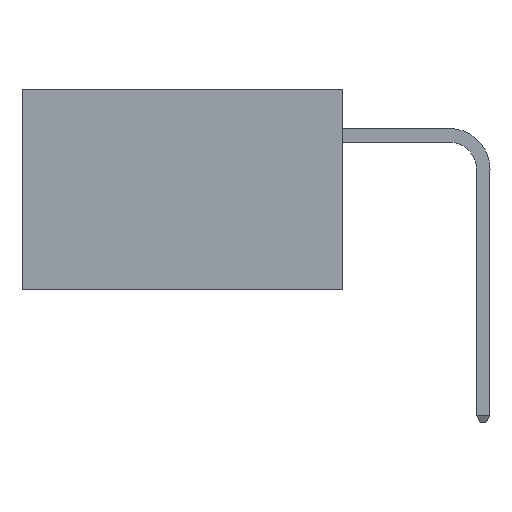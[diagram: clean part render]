
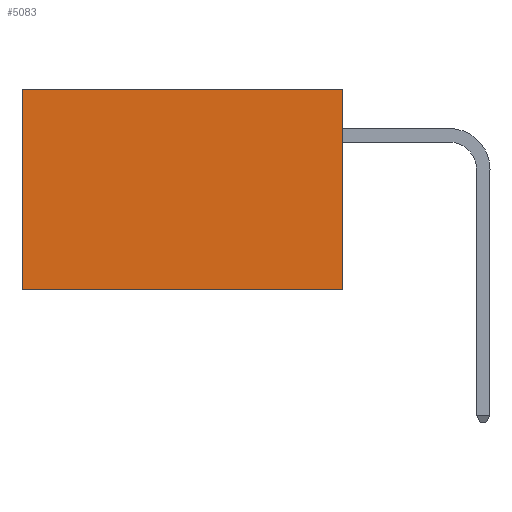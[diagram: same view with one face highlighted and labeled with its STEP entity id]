
A CAD part, left-side view. The second image highlights one B-rep face of the part: STEP entity #5083.
In plain terms, the highlighted planar face has unit normal (-1, 0, 0).
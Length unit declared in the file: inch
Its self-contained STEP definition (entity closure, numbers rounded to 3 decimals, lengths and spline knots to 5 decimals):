
#174 = EDGE_CURVE ( 'NONE', #609, #670, #7226, .T. ) ;
#541 = CARTESIAN_POINT ( 'NONE',  ( 0.277, 0.59, -0.37 ) ) ;
#609 = VERTEX_POINT ( 'NONE', #4975 ) ;
#670 = VERTEX_POINT ( 'NONE', #541 ) ;
#746 = CARTESIAN_POINT ( 'NONE',  ( 0.277, 0.59, 0. ) ) ;
#765 = VECTOR ( 'NONE', #3871, 39.37008 ) ;
#903 = VECTOR ( 'NONE', #4530, 39.37008 ) ;
#1055 = LINE ( 'NONE', #4106, #765 ) ;
#1238 = VERTEX_POINT ( 'NONE', #746 ) ;
#1301 = EDGE_CURVE ( 'NONE', #1238, #670, #5720, .T. ) ;
#1304 = DIRECTION ( 'NONE',  ( 0., 1., 0. ) ) ;
#1619 = CARTESIAN_POINT ( 'NONE',  ( 0.277, 0., -0.37 ) ) ;
#2228 = FACE_OUTER_BOUND ( 'NONE', #5264, .T. ) ;
#2699 = ORIENTED_EDGE ( 'NONE', *, *, #174, .F. ) ;
#2863 = PLANE ( 'NONE',  #5233 ) ;
#2894 = VECTOR ( 'NONE', #1304, 39.37008 ) ;
#2912 = CARTESIAN_POINT ( 'NONE',  ( 0.277, 0., -0.37 ) ) ;
#2942 = VERTEX_POINT ( 'NONE', #5591 ) ;
#3137 = DIRECTION ( 'NONE',  ( 0., 0., -1. ) ) ;
#3151 = DIRECTION ( 'NONE',  ( 1., 0., 0. ) ) ;
#3605 = CARTESIAN_POINT ( 'NONE',  ( 0.277, 0., 0. ) ) ;
#3871 = DIRECTION ( 'NONE',  ( 0., 0., -1. ) ) ;
#4106 = CARTESIAN_POINT ( 'NONE',  ( 0.277, 0., -0.37 ) ) ;
#4530 = DIRECTION ( 'NONE',  ( 0., 1., 0. ) ) ;
#4975 = CARTESIAN_POINT ( 'NONE',  ( 0.277, 0., -0.37 ) ) ;
#4982 = ORIENTED_EDGE ( 'NONE', *, *, #8288, .F. ) ;
#5048 = CARTESIAN_POINT ( 'NONE',  ( 0.277, 0.59, -0.37 ) ) ;
#5083 = ADVANCED_FACE ( 'NONE', ( #2228 ), #2863, .F. ) ;
#5233 = AXIS2_PLACEMENT_3D ( 'NONE', #2912, #3151, #3137 ) ;
#5264 = EDGE_LOOP ( 'NONE', ( #6788, #2699, #4982, #8992 ) ) ;
#5591 = CARTESIAN_POINT ( 'NONE',  ( 0.277, 0., 0. ) ) ;
#5720 = LINE ( 'NONE', #5048, #10040 ) ;
#6788 = ORIENTED_EDGE ( 'NONE', *, *, #1301, .T. ) ;
#7226 = LINE ( 'NONE', #1619, #2894 ) ;
#7616 = LINE ( 'NONE', #3605, #903 ) ;
#8288 = EDGE_CURVE ( 'NONE', #2942, #609, #1055, .T. ) ;
#8718 = EDGE_CURVE ( 'NONE', #2942, #1238, #7616, .T. ) ;
#8992 = ORIENTED_EDGE ( 'NONE', *, *, #8718, .T. ) ;
#9976 = DIRECTION ( 'NONE',  ( 0., 0., -1. ) ) ;
#10040 = VECTOR ( 'NONE', #9976, 39.37008 ) ;
